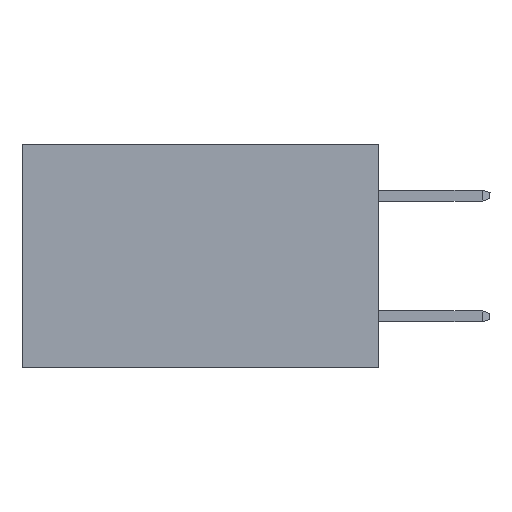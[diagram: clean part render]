
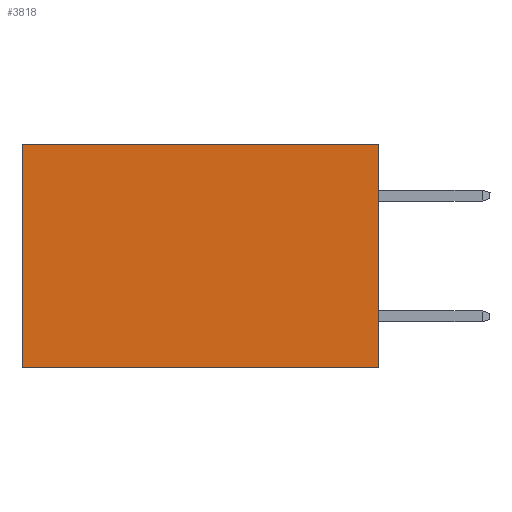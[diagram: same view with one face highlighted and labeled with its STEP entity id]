
A CAD part, left-side view. The second image highlights one B-rep face of the part: STEP entity #3818.
In plain terms, the highlighted planar face has unit normal (-1, 0, 0).
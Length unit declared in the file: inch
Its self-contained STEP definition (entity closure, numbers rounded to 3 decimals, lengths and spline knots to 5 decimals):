
#24 = EDGE_CURVE ( 'NONE', #3727, #9648, #6900, .T. ) ;
#497 = VERTEX_POINT ( 'NONE', #3189 ) ;
#902 = LINE ( 'NONE', #9351, #9973 ) ;
#936 = DIRECTION ( 'NONE',  ( 0., 1., 0. ) ) ;
#977 = CARTESIAN_POINT ( 'NONE',  ( 0.277, 0., -0.37 ) ) ;
#992 = EDGE_LOOP ( 'NONE', ( #4557, #6091, #5930, #7131 ) ) ;
#1048 = VECTOR ( 'NONE', #10182, 39.37008 ) ;
#1452 = DIRECTION ( 'NONE',  ( 0., 0., -1. ) ) ;
#2526 = VECTOR ( 'NONE', #936, 39.37008 ) ;
#2677 = DIRECTION ( 'NONE',  ( 0., 1., 0. ) ) ;
#3189 = CARTESIAN_POINT ( 'NONE',  ( 0.277, 0.59, -0.37 ) ) ;
#3461 = EDGE_CURVE ( 'NONE', #8044, #497, #7163, .T. ) ;
#3680 = FACE_OUTER_BOUND ( 'NONE', #992, .T. ) ;
#3727 = VERTEX_POINT ( 'NONE', #8031 ) ;
#3818 = ADVANCED_FACE ( 'NONE', ( #3680 ), #8214, .F. ) ;
#3896 = CARTESIAN_POINT ( 'NONE',  ( 0.277, 0., 0. ) ) ;
#4489 = AXIS2_PLACEMENT_3D ( 'NONE', #9889, #9962, #4776 ) ;
#4557 = ORIENTED_EDGE ( 'NONE', *, *, #5281, .T. ) ;
#4610 = VECTOR ( 'NONE', #2677, 39.37008 ) ;
#4776 = DIRECTION ( 'NONE',  ( 0., 0., -1. ) ) ;
#5281 = EDGE_CURVE ( 'NONE', #9648, #497, #10349, .T. ) ;
#5930 = ORIENTED_EDGE ( 'NONE', *, *, #8860, .F. ) ;
#6091 = ORIENTED_EDGE ( 'NONE', *, *, #3461, .F. ) ;
#6900 = LINE ( 'NONE', #3896, #4610 ) ;
#7131 = ORIENTED_EDGE ( 'NONE', *, *, #24, .T. ) ;
#7163 = LINE ( 'NONE', #977, #2526 ) ;
#8031 = CARTESIAN_POINT ( 'NONE',  ( 0.277, 0., 0. ) ) ;
#8044 = VERTEX_POINT ( 'NONE', #11099 ) ;
#8214 = PLANE ( 'NONE',  #4489 ) ;
#8297 = CARTESIAN_POINT ( 'NONE',  ( 0.277, 0.59, 0. ) ) ;
#8860 = EDGE_CURVE ( 'NONE', #3727, #8044, #902, .T. ) ;
#9348 = CARTESIAN_POINT ( 'NONE',  ( 0.277, 0.59, -0.37 ) ) ;
#9351 = CARTESIAN_POINT ( 'NONE',  ( 0.277, 0., -0.37 ) ) ;
#9648 = VERTEX_POINT ( 'NONE', #8297 ) ;
#9889 = CARTESIAN_POINT ( 'NONE',  ( 0.277, 0., -0.37 ) ) ;
#9962 = DIRECTION ( 'NONE',  ( 1., 0., 0. ) ) ;
#9973 = VECTOR ( 'NONE', #1452, 39.37008 ) ;
#10182 = DIRECTION ( 'NONE',  ( 0., 0., -1. ) ) ;
#10349 = LINE ( 'NONE', #9348, #1048 ) ;
#11099 = CARTESIAN_POINT ( 'NONE',  ( 0.277, 0., -0.37 ) ) ;
